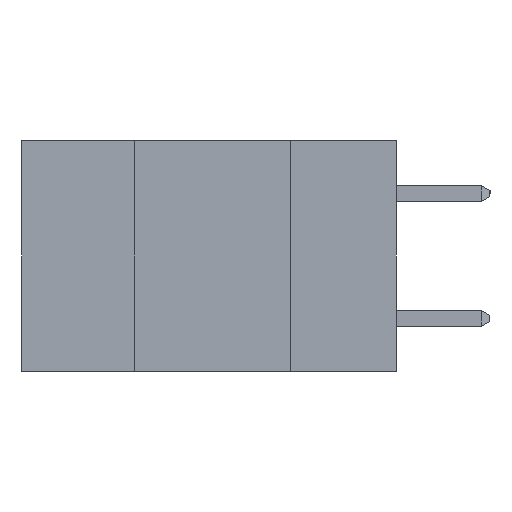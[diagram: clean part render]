
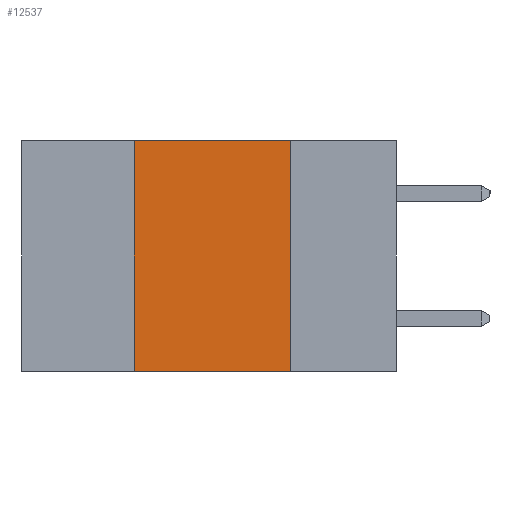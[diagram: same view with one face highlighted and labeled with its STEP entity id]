
A CAD part, left-side view. The second image highlights one B-rep face of the part: STEP entity #12537.
In plain terms, the highlighted planar face has unit normal (-1, 0, 0).
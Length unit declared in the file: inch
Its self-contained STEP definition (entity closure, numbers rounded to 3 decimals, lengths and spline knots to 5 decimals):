
#1080 = EDGE_CURVE ( 'NONE', #4124, #10366, #10530, .T. ) ;
#1217 = DIRECTION ( 'NONE',  ( 0., 0., 1. ) ) ;
#1466 = EDGE_LOOP ( 'NONE', ( #17065, #13566, #10147, #10502 ) ) ;
#1908 = VECTOR ( 'NONE', #1217, 39.37008 ) ;
#2340 = LINE ( 'NONE', #5036, #1908 ) ;
#2706 = FACE_OUTER_BOUND ( 'NONE', #1466, .T. ) ;
#2874 = VERTEX_POINT ( 'NONE', #8944 ) ;
#3025 = VECTOR ( 'NONE', #10301, 39.37008 ) ;
#3703 = CARTESIAN_POINT ( 'NONE',  ( 0., 0.6, 0. ) ) ;
#4124 = VERTEX_POINT ( 'NONE', #4166 ) ;
#4166 = CARTESIAN_POINT ( 'NONE',  ( 0., 0.17, 0. ) ) ;
#4821 = DIRECTION ( 'NONE',  ( 1., 0., 0. ) ) ;
#4998 = CARTESIAN_POINT ( 'NONE',  ( 0., 0.17, -0.37 ) ) ;
#5036 = CARTESIAN_POINT ( 'NONE',  ( 0., 0.42, -0.37 ) ) ;
#6719 = CARTESIAN_POINT ( 'NONE',  ( 0., 0.17, -0.37 ) ) ;
#7596 = DIRECTION ( 'NONE',  ( 0., 0., -1. ) ) ;
#7677 = CARTESIAN_POINT ( 'NONE',  ( 0., 0.42, 0. ) ) ;
#8944 = CARTESIAN_POINT ( 'NONE',  ( 0., 0.42, -0.37 ) ) ;
#9207 = PLANE ( 'NONE',  #12433 ) ;
#10100 = LINE ( 'NONE', #12806, #13658 ) ;
#10147 = ORIENTED_EDGE ( 'NONE', *, *, #16173, .F. ) ;
#10301 = DIRECTION ( 'NONE',  ( 0., -1., 0. ) ) ;
#10366 = VERTEX_POINT ( 'NONE', #6719 ) ;
#10502 = ORIENTED_EDGE ( 'NONE', *, *, #10617, .T. ) ;
#10514 = CARTESIAN_POINT ( 'NONE',  ( 0., 0.6, 0. ) ) ;
#10530 = LINE ( 'NONE', #4998, #11093 ) ;
#10617 = EDGE_CURVE ( 'NONE', #2874, #10366, #10100, .T. ) ;
#11093 = VECTOR ( 'NONE', #15791, 39.37008 ) ;
#11436 = LINE ( 'NONE', #3703, #3025 ) ;
#12433 = AXIS2_PLACEMENT_3D ( 'NONE', #10514, #4821, #7596 ) ;
#12537 = ADVANCED_FACE ( 'NONE', ( #2706 ), #9207, .F. ) ;
#12806 = CARTESIAN_POINT ( 'NONE',  ( 0., 0.6, -0.37 ) ) ;
#13566 = ORIENTED_EDGE ( 'NONE', *, *, #14708, .F. ) ;
#13658 = VECTOR ( 'NONE', #16592, 39.37008 ) ;
#14285 = VERTEX_POINT ( 'NONE', #7677 ) ;
#14708 = EDGE_CURVE ( 'NONE', #14285, #4124, #11436, .T. ) ;
#15791 = DIRECTION ( 'NONE',  ( 0., 0., -1. ) ) ;
#16173 = EDGE_CURVE ( 'NONE', #2874, #14285, #2340, .T. ) ;
#16592 = DIRECTION ( 'NONE',  ( 0., -1., 0. ) ) ;
#17065 = ORIENTED_EDGE ( 'NONE', *, *, #1080, .F. ) ;
